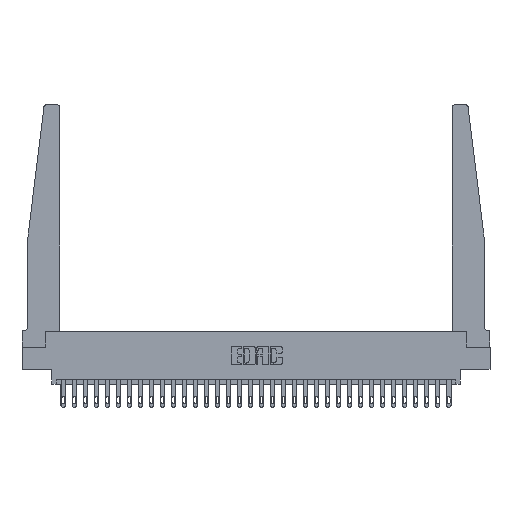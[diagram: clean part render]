
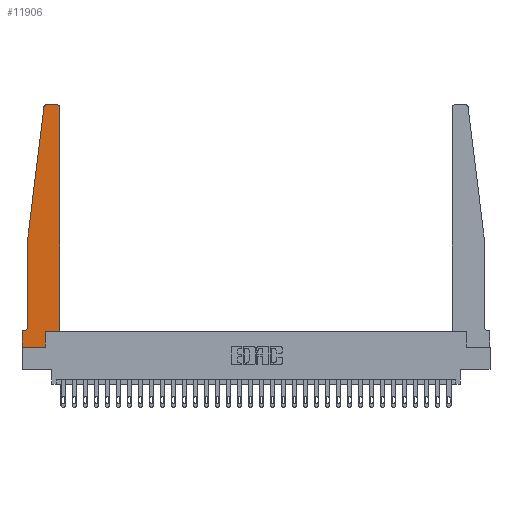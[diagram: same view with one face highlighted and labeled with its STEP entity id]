
A CAD part, top view. The second image highlights one B-rep face of the part: STEP entity #11906.
In plain terms, the highlighted planar face has unit normal (0, 0, 1).
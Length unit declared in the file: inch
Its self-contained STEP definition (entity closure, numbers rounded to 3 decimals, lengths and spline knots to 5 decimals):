
#45 = CARTESIAN_POINT ( 'NONE',  ( 0.425, 0.18, 0.37 ) ) ;
#400 = VERTEX_POINT ( 'NONE', #28337 ) ;
#634 = CARTESIAN_POINT ( 'NONE',  ( 0., 0.1875, 0.37 ) ) ;
#727 = CARTESIAN_POINT ( 'NONE',  ( 0.015, 0.2375, 0.37 ) ) ;
#765 = ORIENTED_EDGE ( 'NONE', *, *, #14217, .T. ) ;
#836 = VECTOR ( 'NONE', #11075, 39.37008 ) ;
#896 = LINE ( 'NONE', #9578, #12819 ) ;
#1033 = PLANE ( 'NONE',  #13217 ) ;
#1179 = DIRECTION ( 'NONE',  ( 1., 0., 0. ) ) ;
#1680 = CARTESIAN_POINT ( 'NONE',  ( 0.065, 1.25, 0.37 ) ) ;
#1998 = CARTESIAN_POINT ( 'NONE',  ( 0.2605, 0.18, 0.37 ) ) ;
#2277 = LINE ( 'NONE', #45, #11218 ) ;
#2617 = DIRECTION ( 'NONE',  ( 1., 0., 0. ) ) ;
#2646 = DIRECTION ( 'NONE',  ( 1., 0., 0. ) ) ;
#2764 = CARTESIAN_POINT ( 'NONE',  ( 0.015, 0.1875, 0.37 ) ) ;
#4105 = ORIENTED_EDGE ( 'NONE', *, *, #10220, .T. ) ;
#4469 = CARTESIAN_POINT ( 'NONE',  ( 0.395, 2.72, 0.37 ) ) ;
#4917 = DIRECTION ( 'NONE',  ( 0., 0., 1. ) ) ;
#5461 = EDGE_CURVE ( 'NONE', #21332, #19720, #18798, .T. ) ;
#5649 = AXIS2_PLACEMENT_3D ( 'NONE', #727, #9869, #28587 ) ;
#5981 = LINE ( 'NONE', #8829, #10431 ) ;
#6132 = VERTEX_POINT ( 'NONE', #28642 ) ;
#6152 = DIRECTION ( 'NONE',  ( -1., 0., 0. ) ) ;
#6193 = LINE ( 'NONE', #12782, #13282 ) ;
#6329 = EDGE_CURVE ( 'NONE', #19720, #13521, #2277, .T. ) ;
#6334 = EDGE_LOOP ( 'NONE', ( #26100, #17063, #765, #10023, #28397, #11200, #23228, #4105, #8650, #7869, #26538, #13454 ) ) ;
#7869 = ORIENTED_EDGE ( 'NONE', *, *, #5461, .T. ) ;
#7932 = AXIS2_PLACEMENT_3D ( 'NONE', #11680, #11542, #20626 ) ;
#8274 = DIRECTION ( 'NONE',  ( 0., -1., 0. ) ) ;
#8650 = ORIENTED_EDGE ( 'NONE', *, *, #10550, .T. ) ;
#8829 = CARTESIAN_POINT ( 'NONE',  ( 0.065, 0.1875, 0.37 ) ) ;
#8922 = VECTOR ( 'NONE', #23050, 39.37008 ) ;
#9107 = VERTEX_POINT ( 'NONE', #20354 ) ;
#9515 = CARTESIAN_POINT ( 'NONE',  ( 0.425, 0.18, 0.37 ) ) ;
#9578 = CARTESIAN_POINT ( 'NONE',  ( 0.065, 1.25, 0.37 ) ) ;
#9756 = LINE ( 'NONE', #18471, #27116 ) ;
#9869 = DIRECTION ( 'NONE',  ( 0., 0., -1. ) ) ;
#9870 = LINE ( 'NONE', #18433, #8922 ) ;
#10023 = ORIENTED_EDGE ( 'NONE', *, *, #23311, .T. ) ;
#10175 = DIRECTION ( 'NONE',  ( 0., 0., 1. ) ) ;
#10220 = EDGE_CURVE ( 'NONE', #400, #18108, #9756, .T. ) ;
#10423 = VERTEX_POINT ( 'NONE', #15603 ) ;
#10431 = VECTOR ( 'NONE', #6152, 39.37008 ) ;
#10550 = EDGE_CURVE ( 'NONE', #18108, #21332, #9870, .T. ) ;
#11075 = DIRECTION ( 'NONE',  ( -1., 0., 0. ) ) ;
#11200 = ORIENTED_EDGE ( 'NONE', *, *, #19831, .T. ) ;
#11214 = CARTESIAN_POINT ( 'NONE',  ( 0.25, 2.75, 0.37 ) ) ;
#11218 = VECTOR ( 'NONE', #18313, 39.37008 ) ;
#11404 = CARTESIAN_POINT ( 'NONE',  ( 0.065, 1.25, 0.37 ) ) ;
#11542 = DIRECTION ( 'NONE',  ( 0., 0., 1. ) ) ;
#11680 = CARTESIAN_POINT ( 'NONE',  ( 0.27653, 2.72, 0.37 ) ) ;
#11906 = ADVANCED_FACE ( 'NONE', ( #23957 ), #1033, .T. ) ;
#12782 = CARTESIAN_POINT ( 'NONE',  ( 0., 0., 0.37 ) ) ;
#12819 = VECTOR ( 'NONE', #18721, 39.37008 ) ;
#13217 = AXIS2_PLACEMENT_3D ( 'NONE', #16917, #10175, #1179 ) ;
#13282 = VECTOR ( 'NONE', #8274, 39.37008 ) ;
#13454 = ORIENTED_EDGE ( 'NONE', *, *, #20075, .T. ) ;
#13521 = VERTEX_POINT ( 'NONE', #27831 ) ;
#14077 = DIRECTION ( 'NONE',  ( -0.122, -0.992, 0. ) ) ;
#14217 = EDGE_CURVE ( 'NONE', #10423, #25911, #27438, .T. ) ;
#14266 = VECTOR ( 'NONE', #14077, 39.37008 ) ;
#15295 = VERTEX_POINT ( 'NONE', #2764 ) ;
#15603 = CARTESIAN_POINT ( 'NONE',  ( 0.24675, 2.72367, 0.37 ) ) ;
#16566 = CIRCLE ( 'NONE', #7932, 0.03 ) ;
#16917 = CARTESIAN_POINT ( 'NONE',  ( 0., 0.1875, 0.37 ) ) ;
#17036 = CARTESIAN_POINT ( 'NONE',  ( 0.395, 2.75, 0.37 ) ) ;
#17062 = EDGE_CURVE ( 'NONE', #9107, #10423, #16566, .T. ) ;
#17063 = ORIENTED_EDGE ( 'NONE', *, *, #17062, .T. ) ;
#17199 = VERTEX_POINT ( 'NONE', #634 ) ;
#17676 = VECTOR ( 'NONE', #2617, 39.37008 ) ;
#18108 = VERTEX_POINT ( 'NONE', #25947 ) ;
#18313 = DIRECTION ( 'NONE',  ( 0., 1., 0. ) ) ;
#18433 = CARTESIAN_POINT ( 'NONE',  ( 0.2605, 0.18, 0.37 ) ) ;
#18471 = CARTESIAN_POINT ( 'NONE',  ( 0., 0., 0.37 ) ) ;
#18589 = CIRCLE ( 'NONE', #28554, 0.03 ) ;
#18721 = DIRECTION ( 'NONE',  ( 0., -1., 0. ) ) ;
#18798 = LINE ( 'NONE', #9515, #17676 ) ;
#18898 = DIRECTION ( 'NONE',  ( 1., 0., 0. ) ) ;
#19295 = CARTESIAN_POINT ( 'NONE',  ( 0.425, 0.18, 0.37 ) ) ;
#19720 = VERTEX_POINT ( 'NONE', #19295 ) ;
#19756 = EDGE_CURVE ( 'NONE', #6132, #15295, #20466, .T. ) ;
#19831 = EDGE_CURVE ( 'NONE', #15295, #17199, #5981, .T. ) ;
#20075 = EDGE_CURVE ( 'NONE', #13521, #24913, #18589, .T. ) ;
#20354 = CARTESIAN_POINT ( 'NONE',  ( 0.27653, 2.75, 0.37 ) ) ;
#20466 = CIRCLE ( 'NONE', #5649, 0.05 ) ;
#20626 = DIRECTION ( 'NONE',  ( 1., 0., 0. ) ) ;
#21332 = VERTEX_POINT ( 'NONE', #1998 ) ;
#23050 = DIRECTION ( 'NONE',  ( 0., 1., 0. ) ) ;
#23102 = EDGE_CURVE ( 'NONE', #17199, #400, #6193, .T. ) ;
#23228 = ORIENTED_EDGE ( 'NONE', *, *, #23102, .T. ) ;
#23311 = EDGE_CURVE ( 'NONE', #25911, #6132, #896, .T. ) ;
#23695 = EDGE_CURVE ( 'NONE', #24913, #9107, #24562, .T. ) ;
#23957 = FACE_OUTER_BOUND ( 'NONE', #6334, .T. ) ;
#24562 = LINE ( 'NONE', #11214, #836 ) ;
#24913 = VERTEX_POINT ( 'NONE', #17036 ) ;
#25911 = VERTEX_POINT ( 'NONE', #1680 ) ;
#25947 = CARTESIAN_POINT ( 'NONE',  ( 0.2605, 0., 0.37 ) ) ;
#26100 = ORIENTED_EDGE ( 'NONE', *, *, #23695, .T. ) ;
#26538 = ORIENTED_EDGE ( 'NONE', *, *, #6329, .T. ) ;
#27116 = VECTOR ( 'NONE', #18898, 39.37008 ) ;
#27438 = LINE ( 'NONE', #11404, #14266 ) ;
#27831 = CARTESIAN_POINT ( 'NONE',  ( 0.425, 2.72, 0.37 ) ) ;
#28337 = CARTESIAN_POINT ( 'NONE',  ( 0., 0., 0.37 ) ) ;
#28397 = ORIENTED_EDGE ( 'NONE', *, *, #19756, .T. ) ;
#28554 = AXIS2_PLACEMENT_3D ( 'NONE', #4469, #4917, #2646 ) ;
#28587 = DIRECTION ( 'NONE',  ( -1., 0., 0. ) ) ;
#28642 = CARTESIAN_POINT ( 'NONE',  ( 0.065, 0.2375, 0.37 ) ) ;
